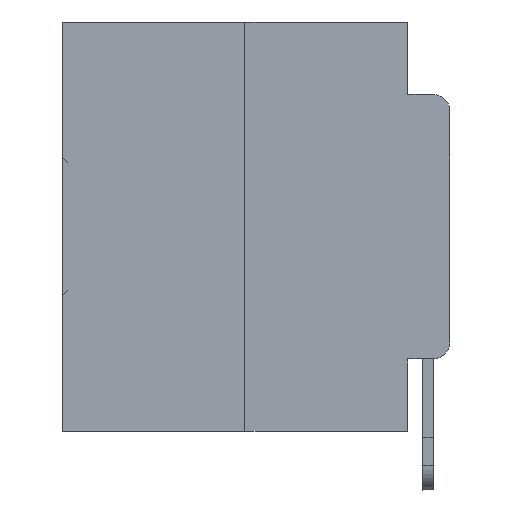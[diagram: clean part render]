
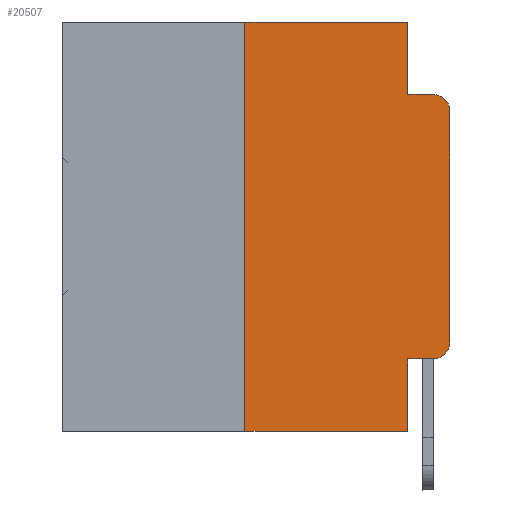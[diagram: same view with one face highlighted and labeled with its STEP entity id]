
A CAD part, left-side view. The second image highlights one B-rep face of the part: STEP entity #20507.
In plain terms, the highlighted planar face has unit normal (-1, 0, 0).
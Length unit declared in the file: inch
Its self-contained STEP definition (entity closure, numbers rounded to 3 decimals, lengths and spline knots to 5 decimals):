
#24 = VECTOR ( 'NONE', #26498, 39.37008 ) ;
#291 = CIRCLE ( 'NONE', #24164, 0.02 ) ;
#296 = DIRECTION ( 'NONE',  ( 0., 0., 1. ) ) ;
#307 = EDGE_CURVE ( 'NONE', #14800, #33927, #19242, .T. ) ;
#566 = ORIENTED_EDGE ( 'NONE', *, *, #9903, .F. ) ;
#1018 = CARTESIAN_POINT ( 'NONE',  ( 0., 0., -0.3915 ) ) ;
#1025 = VECTOR ( 'NONE', #9681, 39.37008 ) ;
#1512 = VERTEX_POINT ( 'NONE', #1018 ) ;
#1530 = ORIENTED_EDGE ( 'NONE', *, *, #307, .F. ) ;
#2250 = ORIENTED_EDGE ( 'NONE', *, *, #23180, .F. ) ;
#3227 = EDGE_CURVE ( 'NONE', #10716, #16278, #291, .T. ) ;
#3604 = DIRECTION ( 'NONE',  ( 0., 0., -1. ) ) ;
#5413 = DIRECTION ( 'NONE',  ( 0., 0., -1. ) ) ;
#5884 = CARTESIAN_POINT ( 'NONE',  ( 0., 0.051, -0.0885 ) ) ;
#6993 = DIRECTION ( 'NONE',  ( 0., 0., -1. ) ) ;
#7144 = FACE_OUTER_BOUND ( 'NONE', #15747, .T. ) ;
#7206 = AXIS2_PLACEMENT_3D ( 'NONE', #23286, #20711, #9780 ) ;
#7410 = VERTEX_POINT ( 'NONE', #15598 ) ;
#7754 = DIRECTION ( 'NONE',  ( 0., 0., -1. ) ) ;
#8108 = ORIENTED_EDGE ( 'NONE', *, *, #19078, .F. ) ;
#9077 = ORIENTED_EDGE ( 'NONE', *, *, #27168, .T. ) ;
#9409 = EDGE_CURVE ( 'NONE', #13457, #16278, #25983, .T. ) ;
#9681 = DIRECTION ( 'NONE',  ( 0., -1., 0. ) ) ;
#9780 = DIRECTION ( 'NONE',  ( 0., 0., -1. ) ) ;
#9903 = EDGE_CURVE ( 'NONE', #18034, #7410, #24726, .T. ) ;
#10652 = DIRECTION ( 'NONE',  ( 0., -1., 0. ) ) ;
#10716 = VERTEX_POINT ( 'NONE', #25542 ) ;
#11613 = DIRECTION ( 'NONE',  ( 1., 0., 0. ) ) ;
#11671 = VERTEX_POINT ( 'NONE', #29234 ) ;
#11796 = AXIS2_PLACEMENT_3D ( 'NONE', #19196, #11613, #3604 ) ;
#11801 = ORIENTED_EDGE ( 'NONE', *, *, #3227, .T. ) ;
#12547 = EDGE_CURVE ( 'NONE', #11671, #1512, #18449, .T. ) ;
#13457 = VERTEX_POINT ( 'NONE', #5884 ) ;
#14282 = CARTESIAN_POINT ( 'NONE',  ( 0., 0.25, 0. ) ) ;
#14658 = CARTESIAN_POINT ( 'NONE',  ( 0., 0.473, 0. ) ) ;
#14800 = VERTEX_POINT ( 'NONE', #16660 ) ;
#14873 = CARTESIAN_POINT ( 'NONE',  ( 0., 0.02, -0.1085 ) ) ;
#15174 = VERTEX_POINT ( 'NONE', #34392 ) ;
#15328 = VECTOR ( 'NONE', #296, 39.37008 ) ;
#15598 = CARTESIAN_POINT ( 'NONE',  ( 0., 0.051, 0. ) ) ;
#15747 = EDGE_LOOP ( 'NONE', ( #23701, #11801, #33652, #8108, #566, #2250, #33213, #1530, #9077, #31095 ) ) ;
#15864 = LINE ( 'NONE', #18541, #31247 ) ;
#15915 = DIRECTION ( 'NONE',  ( 0., 0., 1. ) ) ;
#16278 = VERTEX_POINT ( 'NONE', #17852 ) ;
#16660 = CARTESIAN_POINT ( 'NONE',  ( 0., 0.051, -0.4115 ) ) ;
#17593 = CARTESIAN_POINT ( 'NONE',  ( 0., 0.051, -0.0885 ) ) ;
#17852 = CARTESIAN_POINT ( 'NONE',  ( 0., 0.02, -0.0885 ) ) ;
#18034 = VERTEX_POINT ( 'NONE', #14282 ) ;
#18331 = LINE ( 'NONE', #18482, #24 ) ;
#18449 = CIRCLE ( 'NONE', #7206, 0.02 ) ;
#18482 = CARTESIAN_POINT ( 'NONE',  ( 0., 0.051, -0.4115 ) ) ;
#18541 = CARTESIAN_POINT ( 'NONE',  ( 0., 0.051, 0. ) ) ;
#19078 = EDGE_CURVE ( 'NONE', #7410, #13457, #15864, .T. ) ;
#19196 = CARTESIAN_POINT ( 'NONE',  ( 0., 0.473, 0. ) ) ;
#19242 = LINE ( 'NONE', #32255, #31725 ) ;
#20034 = DIRECTION ( 'NONE',  ( 0., -1., 0. ) ) ;
#20360 = DIRECTION ( 'NONE',  ( -1., 0., 0. ) ) ;
#20362 = EDGE_CURVE ( 'NONE', #1512, #10716, #31637, .T. ) ;
#20507 = ADVANCED_FACE ( 'NONE', ( #7144 ), #22009, .F. ) ;
#20711 = DIRECTION ( 'NONE',  ( -1., 0., 0. ) ) ;
#20731 = CARTESIAN_POINT ( 'NONE',  ( 0., 0., 0. ) ) ;
#20761 = LINE ( 'NONE', #26695, #15328 ) ;
#22009 = PLANE ( 'NONE',  #11796 ) ;
#23180 = EDGE_CURVE ( 'NONE', #15174, #18034, #20761, .T. ) ;
#23286 = CARTESIAN_POINT ( 'NONE',  ( 0., 0.02, -0.3915 ) ) ;
#23701 = ORIENTED_EDGE ( 'NONE', *, *, #20362, .T. ) ;
#24164 = AXIS2_PLACEMENT_3D ( 'NONE', #14873, #20360, #6993 ) ;
#24726 = LINE ( 'NONE', #14658, #28032 ) ;
#24819 = VECTOR ( 'NONE', #10652, 39.37008 ) ;
#25542 = CARTESIAN_POINT ( 'NONE',  ( 0., 0., -0.1085 ) ) ;
#25983 = LINE ( 'NONE', #17593, #1025 ) ;
#26467 = LINE ( 'NONE', #29040, #24819 ) ;
#26498 = DIRECTION ( 'NONE',  ( 0., -1., 0. ) ) ;
#26695 = CARTESIAN_POINT ( 'NONE',  ( 0., 0.25, 0. ) ) ;
#27168 = EDGE_CURVE ( 'NONE', #14800, #11671, #18331, .T. ) ;
#28032 = VECTOR ( 'NONE', #20034, 39.37008 ) ;
#29040 = CARTESIAN_POINT ( 'NONE',  ( 0., 0.473, -0.5 ) ) ;
#29234 = CARTESIAN_POINT ( 'NONE',  ( 0., 0.02, -0.4115 ) ) ;
#31095 = ORIENTED_EDGE ( 'NONE', *, *, #12547, .T. ) ;
#31115 = CARTESIAN_POINT ( 'NONE',  ( 0., 0.051, -0.5 ) ) ;
#31247 = VECTOR ( 'NONE', #7754, 39.37008 ) ;
#31637 = LINE ( 'NONE', #20731, #33319 ) ;
#31725 = VECTOR ( 'NONE', #5413, 39.37008 ) ;
#32255 = CARTESIAN_POINT ( 'NONE',  ( 0., 0.051, 0. ) ) ;
#32979 = EDGE_CURVE ( 'NONE', #15174, #33927, #26467, .T. ) ;
#33213 = ORIENTED_EDGE ( 'NONE', *, *, #32979, .T. ) ;
#33319 = VECTOR ( 'NONE', #15915, 39.37008 ) ;
#33652 = ORIENTED_EDGE ( 'NONE', *, *, #9409, .F. ) ;
#33927 = VERTEX_POINT ( 'NONE', #31115 ) ;
#34392 = CARTESIAN_POINT ( 'NONE',  ( 0., 0.25, -0.5 ) ) ;
